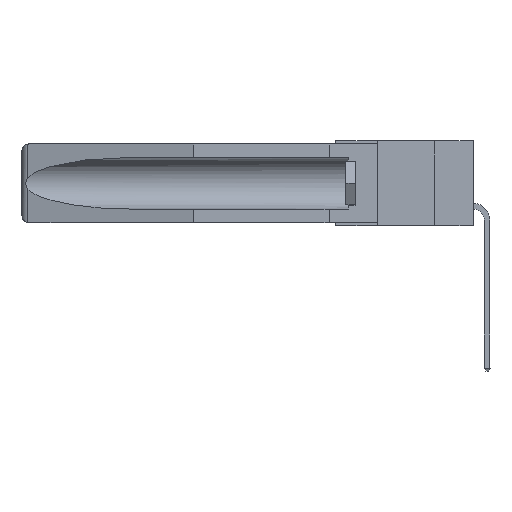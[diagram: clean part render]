
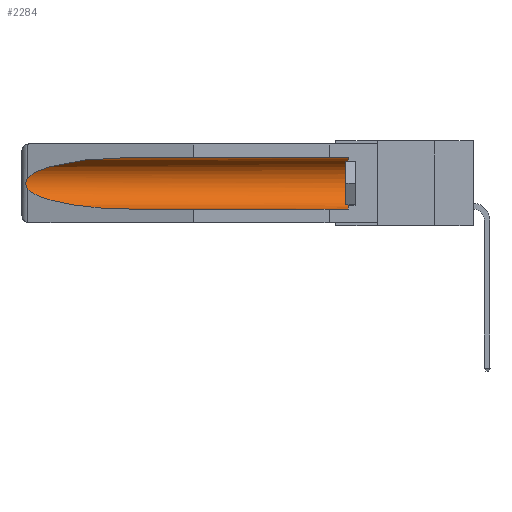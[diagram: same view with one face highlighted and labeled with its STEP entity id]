
A CAD part, left-side view. The second image highlights one B-rep face of the part: STEP entity #2284.
In plain terms, the highlighted cylindrical face has radius 2.857 mm (diameter 5.715 mm), a partial arc.
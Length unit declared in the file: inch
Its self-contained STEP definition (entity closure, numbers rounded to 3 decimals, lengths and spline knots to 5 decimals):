
#159 = EDGE_CURVE ( 'NONE', #1942, #17700, #12307, .T. ) ;
#261 = EDGE_LOOP ( 'NONE', ( #4895, #14054, #5971, #12528, #7571, #6191 ) ) ;
#313 = CARTESIAN_POINT ( 'NONE',  ( 0.155, 1.07973, -0.059 ) ) ;
#466 = VERTEX_POINT ( 'NONE', #524 ) ;
#524 = CARTESIAN_POINT ( 'NONE',  ( 0.26537, 1.52718, -0.14972 ) ) ;
#855 = FACE_OUTER_BOUND ( 'NONE', #261, .T. ) ;
#1634 = VERTEX_POINT ( 'NONE', #15233 ) ;
#1942 = VERTEX_POINT ( 'NONE', #21046 ) ;
#2011 = CYLINDRICAL_SURFACE ( 'NONE', #16632, 0.1125 ) ;
#2284 = ADVANCED_FACE ( 'NONE', ( #855 ), #2011, .F. ) ;
#2296 = CARTESIAN_POINT ( 'NONE',  ( 0.21114, 1.30732, -0.059 ) ) ;
#2306 = EDGE_CURVE ( 'NONE', #17700, #466, #20410, .T. ) ;
#2738 = CARTESIAN_POINT ( 'NONE',  ( 0.155, 0.126, -0.284 ) ) ;
#3309 = VERTEX_POINT ( 'NONE', #2738 ) ;
#3577 = CIRCLE ( 'NONE', #17403, 0.1125 ) ;
#3924 = CARTESIAN_POINT ( 'NONE',  ( 0.26537, 1.52718, -0.14972 ) ) ;
#4184 = CARTESIAN_POINT ( 'NONE',  ( 0.2675, 1.53308, -0.16763 ) ) ;
#4895 = ORIENTED_EDGE ( 'NONE', *, *, #2306, .T. ) ;
#5176 = CARTESIAN_POINT ( 'NONE',  ( 0.155, 1.07973, -0.059 ) ) ;
#5971 = ORIENTED_EDGE ( 'NONE', *, *, #12704, .T. ) ;
#6077 = EDGE_CURVE ( 'NONE', #3309, #1942, #3577, .T. ) ;
#6191 = ORIENTED_EDGE ( 'NONE', *, *, #159, .T. ) ;
#6382 = VERTEX_POINT ( 'NONE', #9251 ) ;
#6432 = CARTESIAN_POINT ( 'NONE',  ( 0.2675, 1.53308, -0.17534 ) ) ;
#7571 = ORIENTED_EDGE ( 'NONE', *, *, #6077, .T. ) ;
#7711 = CARTESIAN_POINT ( 'NONE',  ( 0.2673, 1.5327, -0.16383 ) ) ;
#8131 = CARTESIAN_POINT ( 'NONE',  ( 0.21114, 1.30732, -0.284 ) ) ;
#9015 = B_SPLINE_CURVE_WITH_KNOTS ( 'NONE', 3,
 ( #11161, #10125, #9509, #7711, #4184, #6432, #17203, #10051, #16816, #15563 ),
 .UNSPECIFIED., .F., .F.,
 ( 4, 2, 2, 2, 4 ),
 ( 0., 0.00029, 0.00058, 0.00087, 0.00117 ),
 .UNSPECIFIED. ) ;
#9161 = DIRECTION ( 'NONE',  ( 0., 0., 1. ) ) ;
#9233 = DIRECTION ( 'NONE',  ( 0., 1., 0. ) ) ;
#9251 = CARTESIAN_POINT ( 'NONE',  ( 0.155, 1.07973, -0.284 ) ) ;
#9429 =( BOUNDED_CURVE ( )  B_SPLINE_CURVE ( 3, ( #13546, #10011, #8131, #11721 ),
 .UNSPECIFIED., .F., .F. ) 
 B_SPLINE_CURVE_WITH_KNOTS ( ( 4, 4 ),
 ( 0.1948, 1.5708 ),
 .UNSPECIFIED. ) 
 CURVE ( )  GEOMETRIC_REPRESENTATION_ITEM ( )  RATIONAL_B_SPLINE_CURVE ( ( 1., 0.848, 0.848, 1. ) ) 
 REPRESENTATION_ITEM ( '' )  );
#9509 = CARTESIAN_POINT ( 'NONE',  ( 0.26654, 1.53092, -0.15636 ) ) ;
#10011 = CARTESIAN_POINT ( 'NONE',  ( 0.25451, 1.48313, -0.24835 ) ) ;
#10051 = CARTESIAN_POINT ( 'NONE',  ( 0.26655, 1.53094, -0.18657 ) ) ;
#10125 = CARTESIAN_POINT ( 'NONE',  ( 0.26597, 1.52961, -0.15275 ) ) ;
#10627 = DIRECTION ( 'NONE',  ( 0., -1., 0. ) ) ;
#10744 = VECTOR ( 'NONE', #22368, 39.37008 ) ;
#11011 = LINE ( 'NONE', #20557, #10744 ) ;
#11161 = CARTESIAN_POINT ( 'NONE',  ( 0.26537, 1.52718, -0.14972 ) ) ;
#11721 = CARTESIAN_POINT ( 'NONE',  ( 0.155, 1.07973, -0.284 ) ) ;
#12307 = LINE ( 'NONE', #20340, #17391 ) ;
#12528 = ORIENTED_EDGE ( 'NONE', *, *, #13925, .F. ) ;
#12704 = EDGE_CURVE ( 'NONE', #1634, #6382, #9429, .T. ) ;
#13546 = CARTESIAN_POINT ( 'NONE',  ( 0.26537, 1.52718, -0.19328 ) ) ;
#13925 = EDGE_CURVE ( 'NONE', #3309, #6382, #11011, .T. ) ;
#14054 = ORIENTED_EDGE ( 'NONE', *, *, #21646, .T. ) ;
#14336 = CARTESIAN_POINT ( 'NONE',  ( 0.155, -0.30754, -0.1715 ) ) ;
#15233 = CARTESIAN_POINT ( 'NONE',  ( 0.26537, 1.52718, -0.19328 ) ) ;
#15505 = CARTESIAN_POINT ( 'NONE',  ( 0.155, 0.126, -0.1715 ) ) ;
#15563 = CARTESIAN_POINT ( 'NONE',  ( 0.26537, 1.52718, -0.19328 ) ) ;
#16632 = AXIS2_PLACEMENT_3D ( 'NONE', #14336, #9233, #9161 ) ;
#16816 = CARTESIAN_POINT ( 'NONE',  ( 0.26597, 1.5296, -0.19026 ) ) ;
#17203 = CARTESIAN_POINT ( 'NONE',  ( 0.2673, 1.53269, -0.17917 ) ) ;
#17391 = VECTOR ( 'NONE', #22299, 39.37008 ) ;
#17403 = AXIS2_PLACEMENT_3D ( 'NONE', #15505, #10627, #21244 ) ;
#17700 = VERTEX_POINT ( 'NONE', #5176 ) ;
#20340 = CARTESIAN_POINT ( 'NONE',  ( 0.155, -0.30754, -0.059 ) ) ;
#20410 =( BOUNDED_CURVE ( )  B_SPLINE_CURVE ( 3, ( #313, #2296, #21986, #3924 ),
 .UNSPECIFIED., .F., .T. ) 
 B_SPLINE_CURVE_WITH_KNOTS ( ( 4, 4 ),
 ( 4.71239, 6.08839 ),
 .UNSPECIFIED. ) 
 CURVE ( )  GEOMETRIC_REPRESENTATION_ITEM ( )  RATIONAL_B_SPLINE_CURVE ( ( 1., 0.848, 0.848, 1. ) ) 
 REPRESENTATION_ITEM ( '' )  );
#20557 = CARTESIAN_POINT ( 'NONE',  ( 0.155, -0.30754, -0.284 ) ) ;
#21046 = CARTESIAN_POINT ( 'NONE',  ( 0.155, 0.126, -0.059 ) ) ;
#21244 = DIRECTION ( 'NONE',  ( 0., 0., 1. ) ) ;
#21646 = EDGE_CURVE ( 'NONE', #466, #1634, #9015, .T. ) ;
#21986 = CARTESIAN_POINT ( 'NONE',  ( 0.25451, 1.48313, -0.09465 ) ) ;
#22299 = DIRECTION ( 'NONE',  ( 0., 1., 0. ) ) ;
#22368 = DIRECTION ( 'NONE',  ( 0., 1., 0. ) ) ;
